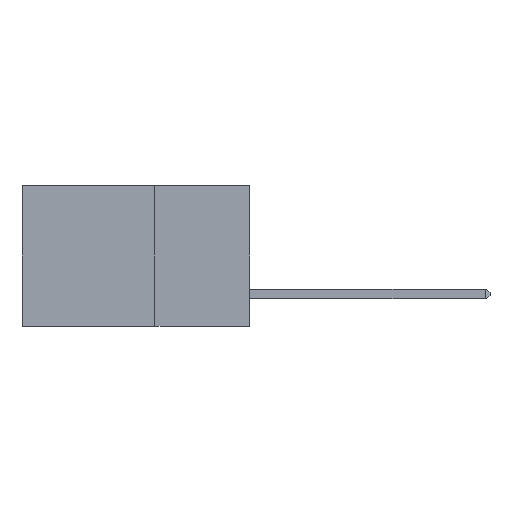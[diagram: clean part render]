
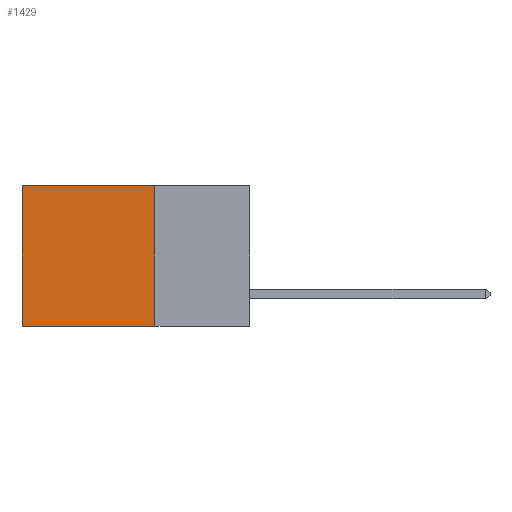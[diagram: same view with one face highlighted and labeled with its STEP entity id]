
A CAD part, left-side view. The second image highlights one B-rep face of the part: STEP entity #1429.
In plain terms, the highlighted planar face has unit normal (-1, 0, 0).
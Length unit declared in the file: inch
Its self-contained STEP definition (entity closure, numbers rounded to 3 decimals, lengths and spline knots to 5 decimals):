
#21 = EDGE_LOOP ( 'NONE', ( #17814, #9737, #31784, #5590 ) ) ;
#1429 = ADVANCED_FACE ( 'NONE', ( #5467 ), #20103, .F. ) ;
#2135 = CARTESIAN_POINT ( 'NONE',  ( 0.2875, 0.6, -0.37 ) ) ;
#2229 = EDGE_CURVE ( 'NONE', #23657, #29286, #7101, .T. ) ;
#3125 = EDGE_CURVE ( 'NONE', #3257, #23657, #25922, .T. ) ;
#3257 = VERTEX_POINT ( 'NONE', #14635 ) ;
#3681 = CARTESIAN_POINT ( 'NONE',  ( 0.2875, 0.25, 0. ) ) ;
#5467 = FACE_OUTER_BOUND ( 'NONE', #21, .T. ) ;
#5590 = ORIENTED_EDGE ( 'NONE', *, *, #3125, .T. ) ;
#6430 = VECTOR ( 'NONE', #23760, 39.37008 ) ;
#6845 = AXIS2_PLACEMENT_3D ( 'NONE', #9881, #27795, #12464 ) ;
#7101 = LINE ( 'NONE', #7662, #26769 ) ;
#7477 = CARTESIAN_POINT ( 'NONE',  ( 0.2875, 0.25, -0.37 ) ) ;
#7662 = CARTESIAN_POINT ( 'NONE',  ( 0.2875, 0.6, 0. ) ) ;
#9737 = ORIENTED_EDGE ( 'NONE', *, *, #22960, .F. ) ;
#9881 = CARTESIAN_POINT ( 'NONE',  ( 0.2875, 0.25, 0. ) ) ;
#10825 = VERTEX_POINT ( 'NONE', #22172 ) ;
#12296 = VECTOR ( 'NONE', #19207, 39.37008 ) ;
#12464 = DIRECTION ( 'NONE',  ( 0., 0., -1. ) ) ;
#14635 = CARTESIAN_POINT ( 'NONE',  ( 0.2875, 0.25, 0. ) ) ;
#15145 = VECTOR ( 'NONE', #25449, 39.37008 ) ;
#17799 = EDGE_CURVE ( 'NONE', #3257, #10825, #20158, .T. ) ;
#17814 = ORIENTED_EDGE ( 'NONE', *, *, #2229, .T. ) ;
#19207 = DIRECTION ( 'NONE',  ( 0., 1., 0. ) ) ;
#20103 = PLANE ( 'NONE',  #6845 ) ;
#20158 = LINE ( 'NONE', #26342, #6430 ) ;
#22172 = CARTESIAN_POINT ( 'NONE',  ( 0.2875, 0.25, -0.37 ) ) ;
#22960 = EDGE_CURVE ( 'NONE', #10825, #29286, #27931, .T. ) ;
#23254 = CARTESIAN_POINT ( 'NONE',  ( 0.2875, 0.6, 0. ) ) ;
#23657 = VERTEX_POINT ( 'NONE', #23254 ) ;
#23760 = DIRECTION ( 'NONE',  ( 0., 0., -1. ) ) ;
#25449 = DIRECTION ( 'NONE',  ( 0., 1., 0. ) ) ;
#25922 = LINE ( 'NONE', #3681, #12296 ) ;
#26342 = CARTESIAN_POINT ( 'NONE',  ( 0.2875, 0.25, 0. ) ) ;
#26769 = VECTOR ( 'NONE', #33326, 39.37008 ) ;
#27795 = DIRECTION ( 'NONE',  ( 1., 0., 0. ) ) ;
#27931 = LINE ( 'NONE', #7477, #15145 ) ;
#29286 = VERTEX_POINT ( 'NONE', #2135 ) ;
#31784 = ORIENTED_EDGE ( 'NONE', *, *, #17799, .F. ) ;
#33326 = DIRECTION ( 'NONE',  ( 0., 0., -1. ) ) ;
